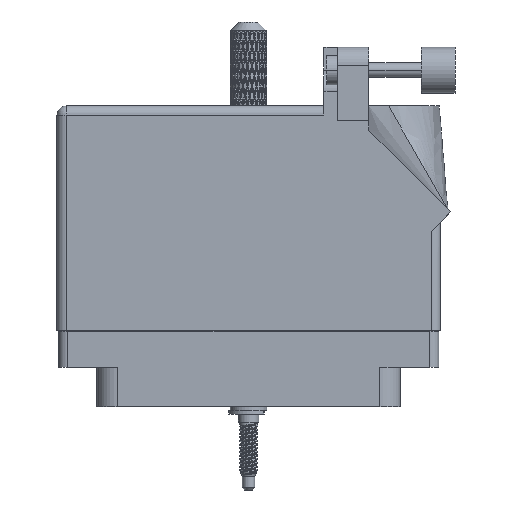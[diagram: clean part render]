
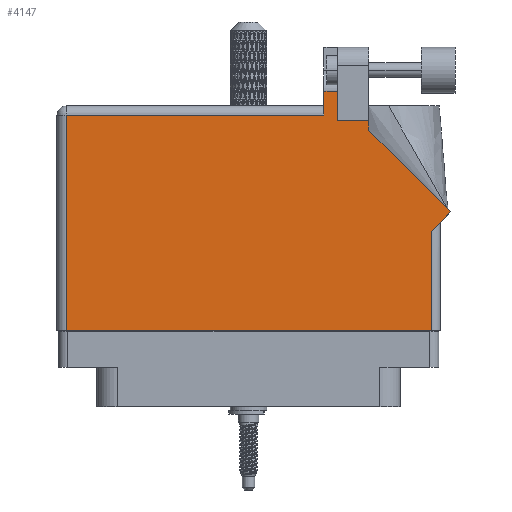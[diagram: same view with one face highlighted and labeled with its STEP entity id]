
A CAD part, front view. The second image highlights one B-rep face of the part: STEP entity #4147.
In plain terms, the highlighted face is planar.
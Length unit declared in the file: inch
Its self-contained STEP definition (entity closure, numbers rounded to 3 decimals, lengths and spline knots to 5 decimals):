
#2116 = ORIENTED_EDGE ( 'NONE', *, *, #87647, .T. ) ;
#2876 = CARTESIAN_POINT ( 'NONE',  ( 0.93777, 1.5315, 0.455 ) ) ;
#4147 = ADVANCED_FACE ( 'NONE', ( #71343 ), #80351, .F. ) ;
#4781 = VERTEX_POINT ( 'NONE', #90556 ) ;
#5726 = CARTESIAN_POINT ( 'NONE',  ( 0.513, 1.43, 0.455 ) ) ;
#6130 = DIRECTION ( 'NONE',  ( -1., 0., 0. ) ) ;
#8513 = EDGE_CURVE ( 'NONE', #4781, #78526, #98189, .T. ) ;
#11143 = CARTESIAN_POINT ( 'NONE',  ( -1.244, -0.1, 0.455 ) ) ;
#17623 = EDGE_CURVE ( 'NONE', #78526, #107799, #75505, .T. ) ;
#19196 = VERTEX_POINT ( 'NONE', #85582 ) ;
#19822 = CARTESIAN_POINT ( 'NONE',  ( 1.37671, 0.70771, 0.455 ) ) ;
#24172 = VECTOR ( 'NONE', #55885, 39.37008 ) ;
#25392 = VECTOR ( 'NONE', #84369, 39.37008 ) ;
#26386 = CARTESIAN_POINT ( 'NONE',  ( 1.244, 0.637, 0.455 ) ) ;
#30356 = CARTESIAN_POINT ( 'NONE',  ( -1.306, 1.368, 0.455 ) ) ;
#30616 = VECTOR ( 'NONE', #65180, 39.37008 ) ;
#31698 = CARTESIAN_POINT ( 'NONE',  ( 0.82, 1.26442, 0.455 ) ) ;
#33943 = ORIENTED_EDGE ( 'NONE', *, *, #62181, .T. ) ;
#34471 = ORIENTED_EDGE ( 'NONE', *, *, #89444, .T. ) ;
#34484 = CARTESIAN_POINT ( 'NONE',  ( -1.306, 1.43, 0.455 ) ) ;
#35733 = DIRECTION ( 'NONE',  ( 1., 0., 0. ) ) ;
#36281 = ORIENTED_EDGE ( 'NONE', *, *, #61658, .T. ) ;
#39916 = EDGE_CURVE ( 'NONE', #60547, #51115, #79783, .T. ) ;
#40955 = DIRECTION ( 'NONE',  ( 0.707, 0.707, 0. ) ) ;
#43651 = LINE ( 'NONE', #2876, #46499 ) ;
#44226 = CARTESIAN_POINT ( 'NONE',  ( 1.244, 0.575, 0.455 ) ) ;
#44930 = VERTEX_POINT ( 'NONE', #81652 ) ;
#46499 = VECTOR ( 'NONE', #90526, 39.37008 ) ;
#46814 = VECTOR ( 'NONE', #102136, 39.37008 ) ;
#48860 = VECTOR ( 'NONE', #35733, 39.37008 ) ;
#49734 = CARTESIAN_POINT ( 'NONE',  ( 1.306, 0.637, 0.455 ) ) ;
#50504 = LINE ( 'NONE', #11143, #30616 ) ;
#51115 = VERTEX_POINT ( 'NONE', #112865 ) ;
#51745 = DIRECTION ( 'NONE',  ( 0., -1., 0. ) ) ;
#51754 = LINE ( 'NONE', #26386, #111739 ) ;
#52962 = DIRECTION ( 'NONE',  ( 0., 1., 0. ) ) ;
#52963 = VERTEX_POINT ( 'NONE', #55918 ) ;
#54007 = EDGE_CURVE ( 'NONE', #44930, #112387, #51754, .T. ) ;
#55885 = DIRECTION ( 'NONE',  ( 0., 1., 0. ) ) ;
#55918 = CARTESIAN_POINT ( 'NONE',  ( 0.513, 1.5315, 0.455 ) ) ;
#56078 = EDGE_LOOP ( 'NONE', ( #34471, #36281, #33943, #100744, #70179, #66056, #118059, #2116, #117058, #93385, #79549 ) ) ;
#59354 = CARTESIAN_POINT ( 'NONE',  ( 0.607, 1.33, 0.455 ) ) ;
#59800 = VECTOR ( 'NONE', #40955, 39.37008 ) ;
#60547 = VERTEX_POINT ( 'NONE', #68007 ) ;
#61658 = EDGE_CURVE ( 'NONE', #19196, #52963, #43651, .T. ) ;
#62181 = EDGE_CURVE ( 'NONE', #52963, #60547, #85047, .T. ) ;
#62318 = DIRECTION ( 'NONE',  ( -1., 0., 0. ) ) ;
#64393 = LINE ( 'NONE', #87411, #94531 ) ;
#65180 = DIRECTION ( 'NONE',  ( 0., -1., 0. ) ) ;
#65873 = EDGE_CURVE ( 'NONE', #105915, #44930, #90404, .T. ) ;
#66056 = ORIENTED_EDGE ( 'NONE', *, *, #65873, .T. ) ;
#68007 = CARTESIAN_POINT ( 'NONE',  ( 0.513, 1.368, 0.455 ) ) ;
#70179 = ORIENTED_EDGE ( 'NONE', *, *, #94056, .T. ) ;
#71162 = LINE ( 'NONE', #101734, #46814 ) ;
#71343 = FACE_OUTER_BOUND ( 'NONE', #56078, .T. ) ;
#71655 = CARTESIAN_POINT ( 'NONE',  ( -1.306, -0.1, 0.455 ) ) ;
#75505 = LINE ( 'NONE', #100715, #24172 ) ;
#78526 = VERTEX_POINT ( 'NONE', #31698 ) ;
#79549 = ORIENTED_EDGE ( 'NONE', *, *, #109333, .T. ) ;
#79578 = DIRECTION ( 'NONE',  ( 0., 0., -1. ) ) ;
#79783 = LINE ( 'NONE', #30356, #95515 ) ;
#80351 = PLANE ( 'NONE',  #95944 ) ;
#81652 = CARTESIAN_POINT ( 'NONE',  ( 1.244, -0.1, 0.455 ) ) ;
#84214 = LINE ( 'NONE', #49734, #59800 ) ;
#84369 = DIRECTION ( 'NONE',  ( -0.707, 0.707, 0. ) ) ;
#85047 = LINE ( 'NONE', #5726, #109221 ) ;
#85582 = CARTESIAN_POINT ( 'NONE',  ( 0.607, 1.5315, 0.455 ) ) ;
#87307 = CARTESIAN_POINT ( 'NONE',  ( -1.244, -0.1, 0.455 ) ) ;
#87411 = CARTESIAN_POINT ( 'NONE',  ( 0.82, 1.33, 0.455 ) ) ;
#87647 = EDGE_CURVE ( 'NONE', #112387, #4781, #84214, .T. ) ;
#89444 = EDGE_CURVE ( 'NONE', #99885, #19196, #71162, .T. ) ;
#90404 = LINE ( 'NONE', #71655, #48860 ) ;
#90526 = DIRECTION ( 'NONE',  ( -1., 0., 0. ) ) ;
#90556 = CARTESIAN_POINT ( 'NONE',  ( 1.37671, 0.70771, 0.455 ) ) ;
#93385 = ORIENTED_EDGE ( 'NONE', *, *, #17623, .T. ) ;
#94056 = EDGE_CURVE ( 'NONE', #51115, #105915, #50504, .T. ) ;
#94531 = VECTOR ( 'NONE', #6130, 39.37008 ) ;
#95515 = VECTOR ( 'NONE', #113935, 39.37008 ) ;
#95944 = AXIS2_PLACEMENT_3D ( 'NONE', #34484, #79578, #62318 ) ;
#98189 = LINE ( 'NONE', #19822, #25392 ) ;
#99885 = VERTEX_POINT ( 'NONE', #59354 ) ;
#100715 = CARTESIAN_POINT ( 'NONE',  ( 0.82, 1.26442, 0.455 ) ) ;
#100744 = ORIENTED_EDGE ( 'NONE', *, *, #39916, .T. ) ;
#101734 = CARTESIAN_POINT ( 'NONE',  ( 0.607, 1.33, 0.455 ) ) ;
#102136 = DIRECTION ( 'NONE',  ( 0., 1., 0. ) ) ;
#105915 = VERTEX_POINT ( 'NONE', #87307 ) ;
#106264 = CARTESIAN_POINT ( 'NONE',  ( 0.82, 1.33, 0.455 ) ) ;
#107799 = VERTEX_POINT ( 'NONE', #106264 ) ;
#109221 = VECTOR ( 'NONE', #51745, 39.37008 ) ;
#109333 = EDGE_CURVE ( 'NONE', #107799, #99885, #64393, .T. ) ;
#111739 = VECTOR ( 'NONE', #52962, 39.37008 ) ;
#112387 = VERTEX_POINT ( 'NONE', #44226 ) ;
#112865 = CARTESIAN_POINT ( 'NONE',  ( -1.244, 1.368, 0.455 ) ) ;
#113935 = DIRECTION ( 'NONE',  ( -1., 0., 0. ) ) ;
#117058 = ORIENTED_EDGE ( 'NONE', *, *, #8513, .T. ) ;
#118059 = ORIENTED_EDGE ( 'NONE', *, *, #54007, .T. ) ;
